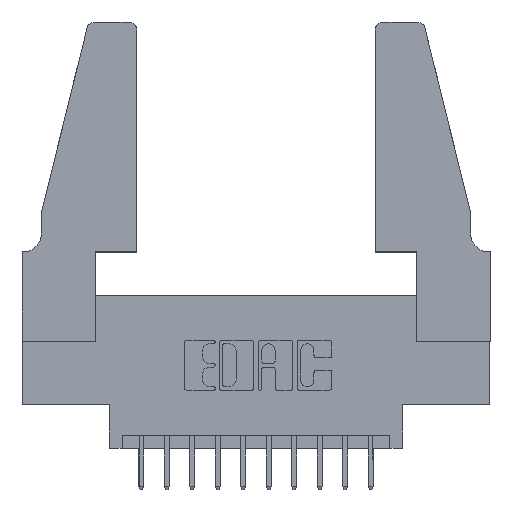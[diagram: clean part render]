
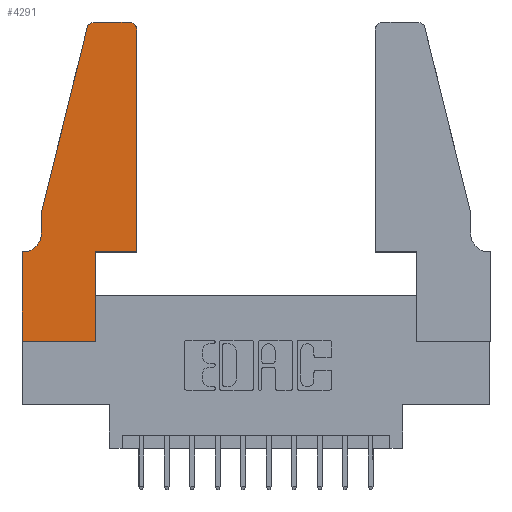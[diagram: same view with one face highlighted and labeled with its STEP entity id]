
A CAD part, top view. The second image highlights one B-rep face of the part: STEP entity #4291.
In plain terms, the highlighted planar face has unit normal (0, 0, 1).
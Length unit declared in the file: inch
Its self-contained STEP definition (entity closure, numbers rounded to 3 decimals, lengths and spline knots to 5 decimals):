
#270 = EDGE_CURVE ( 'NONE', #4250, #10502, #9589, .T. ) ;
#393 = EDGE_CURVE ( 'NONE', #7756, #6575, #5748, .T. ) ;
#784 = LINE ( 'NONE', #8869, #4537 ) ;
#871 = DIRECTION ( 'NONE',  ( 1., 0., 0. ) ) ;
#1027 = EDGE_CURVE ( 'NONE', #3547, #4888, #12545, .T. ) ;
#1045 = CARTESIAN_POINT ( 'NONE',  ( 0.25487, 1.22718, 0.37 ) ) ;
#1261 = CARTESIAN_POINT ( 'NONE',  ( 0.0755, 0.35, 0.37 ) ) ;
#1303 = EDGE_CURVE ( 'NONE', #3533, #3547, #4492, .T. ) ;
#1365 = CIRCLE ( 'NONE', #1605, 0.03 ) ;
#1437 = CIRCLE ( 'NONE', #12643, 0.03 ) ;
#1473 = AXIS2_PLACEMENT_3D ( 'NONE', #3690, #6267, #5039 ) ;
#1492 = CARTESIAN_POINT ( 'NONE',  ( 0.0755, 0.5, 0.37 ) ) ;
#1605 = AXIS2_PLACEMENT_3D ( 'NONE', #7303, #6346, #10699 ) ;
#1910 = CARTESIAN_POINT ( 'NONE',  ( 0., 0., 0.37 ) ) ;
#2103 = DIRECTION ( 'NONE',  ( 1., 0., 0. ) ) ;
#2305 = ORIENTED_EDGE ( 'NONE', *, *, #5501, .T. ) ;
#2564 = DIRECTION ( 'NONE',  ( 0., 1., 0. ) ) ;
#2568 = ORIENTED_EDGE ( 'NONE', *, *, #3381, .T. ) ;
#2711 = VECTOR ( 'NONE', #4080, 39.37008 ) ;
#3052 = DIRECTION ( 'NONE',  ( 1., 0., 0. ) ) ;
#3315 = AXIS2_PLACEMENT_3D ( 'NONE', #6383, #10788, #5226 ) ;
#3381 = EDGE_CURVE ( 'NONE', #11438, #4250, #1437, .T. ) ;
#3421 = CARTESIAN_POINT ( 'NONE',  ( 0., 0.35, 0.37 ) ) ;
#3533 = VERTEX_POINT ( 'NONE', #12327 ) ;
#3540 = ORIENTED_EDGE ( 'NONE', *, *, #1303, .T. ) ;
#3547 = VERTEX_POINT ( 'NONE', #3421 ) ;
#3690 = CARTESIAN_POINT ( 'NONE',  ( 0., 0.35, 0.37 ) ) ;
#3784 = ORIENTED_EDGE ( 'NONE', *, *, #9485, .T. ) ;
#3815 = ORIENTED_EDGE ( 'NONE', *, *, #11712, .T. ) ;
#4080 = DIRECTION ( 'NONE',  ( 0., 1., 0. ) ) ;
#4085 = CARTESIAN_POINT ( 'NONE',  ( 0.4505, 0.35, 0.37 ) ) ;
#4232 = CARTESIAN_POINT ( 'NONE',  ( 0.284, 1.25, 0.37 ) ) ;
#4250 = VERTEX_POINT ( 'NONE', #11658 ) ;
#4291 = ADVANCED_FACE ( 'NONE', ( #14381 ), #7029, .T. ) ;
#4314 = CARTESIAN_POINT ( 'NONE',  ( 0.4205, 1.22, 0.37 ) ) ;
#4394 = VECTOR ( 'NONE', #2564, 39.37008 ) ;
#4492 = LINE ( 'NONE', #1261, #14264 ) ;
#4537 = VECTOR ( 'NONE', #8664, 39.37008 ) ;
#4588 = DIRECTION ( 'NONE',  ( -1., 0., 0. ) ) ;
#4800 = CARTESIAN_POINT ( 'NONE',  ( 0.4505, 0.35, 0.37 ) ) ;
#4888 = VERTEX_POINT ( 'NONE', #4903 ) ;
#4903 = CARTESIAN_POINT ( 'NONE',  ( 0., 0., 0.37 ) ) ;
#5039 = DIRECTION ( 'NONE',  ( 1., 0., 0. ) ) ;
#5226 = DIRECTION ( 'NONE',  ( -1., 0., 0. ) ) ;
#5501 = EDGE_CURVE ( 'NONE', #6575, #12687, #13098, .T. ) ;
#5626 = CARTESIAN_POINT ( 'NONE',  ( 0.4505, 0.35, 0.37 ) ) ;
#5748 = LINE ( 'NONE', #11821, #2711 ) ;
#5928 = DIRECTION ( 'NONE',  ( -0.239, -0.971, 0. ) ) ;
#5948 = CARTESIAN_POINT ( 'NONE',  ( 0.4505, 1.22, 0.37 ) ) ;
#6163 = LINE ( 'NONE', #1492, #10391 ) ;
#6267 = DIRECTION ( 'NONE',  ( 0., 0., 1. ) ) ;
#6346 = DIRECTION ( 'NONE',  ( 0., 0., 1. ) ) ;
#6383 = CARTESIAN_POINT ( 'NONE',  ( 0.0055, 0.42, 0.37 ) ) ;
#6426 = ORIENTED_EDGE ( 'NONE', *, *, #10522, .T. ) ;
#6472 = EDGE_CURVE ( 'NONE', #13700, #14193, #784, .T. ) ;
#6505 = ORIENTED_EDGE ( 'NONE', *, *, #12995, .T. ) ;
#6575 = VERTEX_POINT ( 'NONE', #10235 ) ;
#6934 = ORIENTED_EDGE ( 'NONE', *, *, #6472, .T. ) ;
#7029 = PLANE ( 'NONE',  #1473 ) ;
#7042 = DIRECTION ( 'NONE',  ( -1., 0., 0. ) ) ;
#7141 = VERTEX_POINT ( 'NONE', #1045 ) ;
#7303 = CARTESIAN_POINT ( 'NONE',  ( 0.284, 1.22, 0.37 ) ) ;
#7471 = CARTESIAN_POINT ( 'NONE',  ( 0., 0., 0.37 ) ) ;
#7756 = VERTEX_POINT ( 'NONE', #10905 ) ;
#8136 = CARTESIAN_POINT ( 'NONE',  ( 0.2605, 1.25, 0.37 ) ) ;
#8258 = ORIENTED_EDGE ( 'NONE', *, *, #1027, .T. ) ;
#8664 = DIRECTION ( 'NONE',  ( 0., -1., 0. ) ) ;
#8805 = CARTESIAN_POINT ( 'NONE',  ( 0.0755, 0.5, 0.37 ) ) ;
#8869 = CARTESIAN_POINT ( 'NONE',  ( 0.0755, 0.5, 0.37 ) ) ;
#8959 = LINE ( 'NONE', #4800, #4394 ) ;
#9450 = VECTOR ( 'NONE', #2103, 39.37008 ) ;
#9485 = EDGE_CURVE ( 'NONE', #4888, #7756, #11117, .T. ) ;
#9589 = LINE ( 'NONE', #8136, #13944 ) ;
#9757 = DIRECTION ( 'NONE',  ( 0., -1., 0. ) ) ;
#9876 = CIRCLE ( 'NONE', #3315, 0.07 ) ;
#10235 = CARTESIAN_POINT ( 'NONE',  ( 0.2865, 0.35, 0.37 ) ) ;
#10391 = VECTOR ( 'NONE', #5928, 39.37008 ) ;
#10502 = VERTEX_POINT ( 'NONE', #4232 ) ;
#10522 = EDGE_CURVE ( 'NONE', #14193, #3533, #9876, .T. ) ;
#10686 = EDGE_LOOP ( 'NONE', ( #12269, #6505, #3815, #6934, #6426, #3540, #8258, #3784, #11162, #2305, #11122, #2568 ) ) ;
#10699 = DIRECTION ( 'NONE',  ( 1., 0., 0. ) ) ;
#10756 = VECTOR ( 'NONE', #3052, 39.37008 ) ;
#10788 = DIRECTION ( 'NONE',  ( 0., 0., -1. ) ) ;
#10905 = CARTESIAN_POINT ( 'NONE',  ( 0.2865, 0., 0.37 ) ) ;
#11117 = LINE ( 'NONE', #1910, #10756 ) ;
#11122 = ORIENTED_EDGE ( 'NONE', *, *, #12909, .T. ) ;
#11124 = CARTESIAN_POINT ( 'NONE',  ( 0.0755, 0.42, 0.37 ) ) ;
#11162 = ORIENTED_EDGE ( 'NONE', *, *, #393, .T. ) ;
#11438 = VERTEX_POINT ( 'NONE', #5948 ) ;
#11658 = CARTESIAN_POINT ( 'NONE',  ( 0.4205, 1.25, 0.37 ) ) ;
#11712 = EDGE_CURVE ( 'NONE', #7141, #13700, #6163, .T. ) ;
#11821 = CARTESIAN_POINT ( 'NONE',  ( 0.2865, 0.35, 0.37 ) ) ;
#12187 = VECTOR ( 'NONE', #9757, 39.37008 ) ;
#12269 = ORIENTED_EDGE ( 'NONE', *, *, #270, .T. ) ;
#12327 = CARTESIAN_POINT ( 'NONE',  ( 0.0055, 0.35, 0.37 ) ) ;
#12545 = LINE ( 'NONE', #7471, #12187 ) ;
#12643 = AXIS2_PLACEMENT_3D ( 'NONE', #4314, #13043, #871 ) ;
#12687 = VERTEX_POINT ( 'NONE', #4085 ) ;
#12909 = EDGE_CURVE ( 'NONE', #12687, #11438, #8959, .T. ) ;
#12995 = EDGE_CURVE ( 'NONE', #10502, #7141, #1365, .T. ) ;
#13043 = DIRECTION ( 'NONE',  ( 0., 0., 1. ) ) ;
#13098 = LINE ( 'NONE', #5626, #9450 ) ;
#13700 = VERTEX_POINT ( 'NONE', #8805 ) ;
#13944 = VECTOR ( 'NONE', #7042, 39.37008 ) ;
#14193 = VERTEX_POINT ( 'NONE', #11124 ) ;
#14264 = VECTOR ( 'NONE', #4588, 39.37008 ) ;
#14381 = FACE_OUTER_BOUND ( 'NONE', #10686, .T. ) ;
